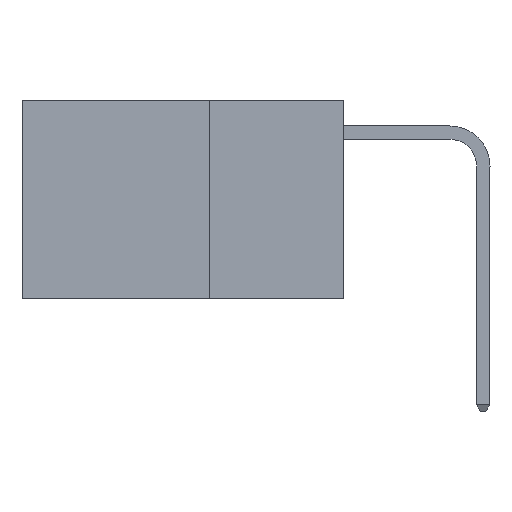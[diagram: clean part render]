
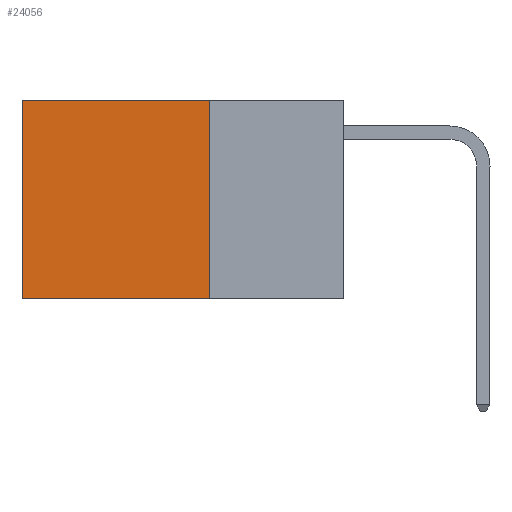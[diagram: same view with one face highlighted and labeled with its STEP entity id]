
A CAD part, left-side view. The second image highlights one B-rep face of the part: STEP entity #24056.
In plain terms, the highlighted planar face has unit normal (-1, 0, 0).
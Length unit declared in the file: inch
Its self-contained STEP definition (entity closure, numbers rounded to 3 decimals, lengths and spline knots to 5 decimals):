
#297 = EDGE_CURVE ( 'NONE', #14158, #783, #23241, .T. ) ;
#783 = VERTEX_POINT ( 'NONE', #14742 ) ;
#837 = ORIENTED_EDGE ( 'NONE', *, *, #22114, .F. ) ;
#1246 = VECTOR ( 'NONE', #10035, 39.37008 ) ;
#1509 = PLANE ( 'NONE',  #8257 ) ;
#3872 = VECTOR ( 'NONE', #4476, 39.37008 ) ;
#4476 = DIRECTION ( 'NONE',  ( 0., 1., 0. ) ) ;
#4841 = CARTESIAN_POINT ( 'NONE',  ( 0.2625, 0.25, 0. ) ) ;
#5049 = LINE ( 'NONE', #13532, #9768 ) ;
#5694 = DIRECTION ( 'NONE',  ( 1., 0., 0. ) ) ;
#6943 = FACE_OUTER_BOUND ( 'NONE', #14071, .T. ) ;
#7384 = LINE ( 'NONE', #14512, #3872 ) ;
#7497 = ORIENTED_EDGE ( 'NONE', *, *, #8047, .T. ) ;
#8031 = CARTESIAN_POINT ( 'NONE',  ( 0.2625, 0.25, 0. ) ) ;
#8047 = EDGE_CURVE ( 'NONE', #9915, #14158, #5049, .T. ) ;
#8257 = AXIS2_PLACEMENT_3D ( 'NONE', #15680, #5694, #19726 ) ;
#9768 = VECTOR ( 'NONE', #15555, 39.37008 ) ;
#9915 = VERTEX_POINT ( 'NONE', #4841 ) ;
#10035 = DIRECTION ( 'NONE',  ( 0., 0., -1. ) ) ;
#10345 = CARTESIAN_POINT ( 'NONE',  ( 0.2625, 0.6, 0. ) ) ;
#10723 = VECTOR ( 'NONE', #24106, 39.37008 ) ;
#12064 = LINE ( 'NONE', #8031, #1246 ) ;
#12207 = ORIENTED_EDGE ( 'NONE', *, *, #297, .T. ) ;
#13532 = CARTESIAN_POINT ( 'NONE',  ( 0.2625, 0.25, 0. ) ) ;
#14071 = EDGE_LOOP ( 'NONE', ( #12207, #21646, #837, #7497 ) ) ;
#14158 = VERTEX_POINT ( 'NONE', #10345 ) ;
#14512 = CARTESIAN_POINT ( 'NONE',  ( 0.2625, 0.25, -0.37 ) ) ;
#14742 = CARTESIAN_POINT ( 'NONE',  ( 0.2625, 0.6, -0.37 ) ) ;
#15555 = DIRECTION ( 'NONE',  ( 0., 1., 0. ) ) ;
#15680 = CARTESIAN_POINT ( 'NONE',  ( 0.2625, 0.25, 0. ) ) ;
#16641 = EDGE_CURVE ( 'NONE', #19865, #783, #7384, .T. ) ;
#19114 = CARTESIAN_POINT ( 'NONE',  ( 0.2625, 0.25, -0.37 ) ) ;
#19726 = DIRECTION ( 'NONE',  ( 0., 0., -1. ) ) ;
#19865 = VERTEX_POINT ( 'NONE', #19114 ) ;
#21646 = ORIENTED_EDGE ( 'NONE', *, *, #16641, .F. ) ;
#22114 = EDGE_CURVE ( 'NONE', #9915, #19865, #12064, .T. ) ;
#23241 = LINE ( 'NONE', #24183, #10723 ) ;
#24056 = ADVANCED_FACE ( 'NONE', ( #6943 ), #1509, .F. ) ;
#24106 = DIRECTION ( 'NONE',  ( 0., 0., -1. ) ) ;
#24183 = CARTESIAN_POINT ( 'NONE',  ( 0.2625, 0.6, 0. ) ) ;
